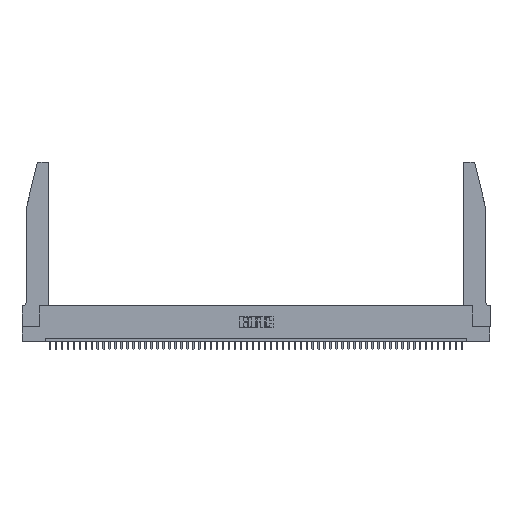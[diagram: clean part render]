
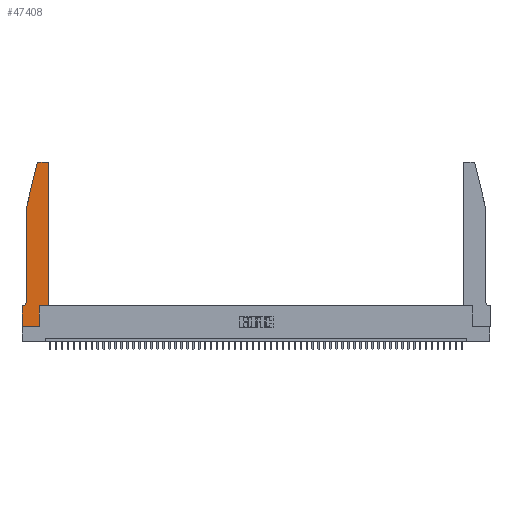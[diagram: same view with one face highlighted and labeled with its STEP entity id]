
A CAD part, top view. The second image highlights one B-rep face of the part: STEP entity #47408.
In plain terms, the highlighted planar face has unit normal (0, 0, 1).
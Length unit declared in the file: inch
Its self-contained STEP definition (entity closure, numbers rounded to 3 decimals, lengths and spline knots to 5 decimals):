
#1088 = VERTEX_POINT ( 'NONE', #7912 ) ;
#1743 = CARTESIAN_POINT ( 'NONE',  ( 0., 0.35, 0.37 ) ) ;
#1959 = VERTEX_POINT ( 'NONE', #51669 ) ;
#2248 = CARTESIAN_POINT ( 'NONE',  ( 0., 0.35, 0.37 ) ) ;
#2281 = CARTESIAN_POINT ( 'NONE',  ( 0.2605, 2.75, 0.37 ) ) ;
#2965 = ORIENTED_EDGE ( 'NONE', *, *, #28072, .T. ) ;
#4232 = VERTEX_POINT ( 'NONE', #18782 ) ;
#4546 = DIRECTION ( 'NONE',  ( -1., 0., 0. ) ) ;
#4662 = ORIENTED_EDGE ( 'NONE', *, *, #48811, .T. ) ;
#4726 = ORIENTED_EDGE ( 'NONE', *, *, #49574, .T. ) ;
#5114 = DIRECTION ( 'NONE',  ( 1., 0., 0. ) ) ;
#5791 = VERTEX_POINT ( 'NONE', #7713 ) ;
#5818 = VECTOR ( 'NONE', #52841, 39.37008 ) ;
#7523 = CARTESIAN_POINT ( 'NONE',  ( 0.4205, 2.75, 0.37 ) ) ;
#7713 = CARTESIAN_POINT ( 'NONE',  ( 0.4505, 2.72, 0.37 ) ) ;
#7912 = CARTESIAN_POINT ( 'NONE',  ( 0., 0., 0.37 ) ) ;
#8651 = LINE ( 'NONE', #51778, #38439 ) ;
#9214 = CARTESIAN_POINT ( 'NONE',  ( 0.25487, 2.72718, 0.37 ) ) ;
#10478 = PLANE ( 'NONE',  #39131 ) ;
#10817 = EDGE_CURVE ( 'NONE', #13678, #48190, #16978, .T. ) ;
#10908 = DIRECTION ( 'NONE',  ( -1., 0., 0. ) ) ;
#12120 = ORIENTED_EDGE ( 'NONE', *, *, #10817, .T. ) ;
#12957 = VERTEX_POINT ( 'NONE', #7523 ) ;
#13678 = VERTEX_POINT ( 'NONE', #21338 ) ;
#14140 = CARTESIAN_POINT ( 'NONE',  ( 0.4505, 0.35, 0.37 ) ) ;
#15595 = ORIENTED_EDGE ( 'NONE', *, *, #46903, .T. ) ;
#15779 = ORIENTED_EDGE ( 'NONE', *, *, #20057, .T. ) ;
#16077 = CARTESIAN_POINT ( 'NONE',  ( 0.4505, 0.35, 0.37 ) ) ;
#16978 = LINE ( 'NONE', #44925, #5818 ) ;
#18343 = VECTOR ( 'NONE', #38082, 39.37008 ) ;
#18782 = CARTESIAN_POINT ( 'NONE',  ( 0.2865, 0.35, 0.37 ) ) ;
#19298 = DIRECTION ( 'NONE',  ( -1., 0., 0. ) ) ;
#20057 = EDGE_CURVE ( 'NONE', #41519, #4232, #24482, .T. ) ;
#20104 = EDGE_CURVE ( 'NONE', #39838, #5791, #31553, .T. ) ;
#21002 = CARTESIAN_POINT ( 'NONE',  ( 0.284, 2.72, 0.37 ) ) ;
#21013 = VERTEX_POINT ( 'NONE', #1743 ) ;
#21338 = CARTESIAN_POINT ( 'NONE',  ( 0.0755, 2., 0.37 ) ) ;
#22242 = ORIENTED_EDGE ( 'NONE', *, *, #29675, .T. ) ;
#23185 = DIRECTION ( 'NONE',  ( 0., 1., 0. ) ) ;
#24482 = LINE ( 'NONE', #29772, #42487 ) ;
#24500 = EDGE_CURVE ( 'NONE', #29545, #13678, #40934, .T. ) ;
#25381 = ORIENTED_EDGE ( 'NONE', *, *, #24500, .T. ) ;
#25647 = ORIENTED_EDGE ( 'NONE', *, *, #41718, .T. ) ;
#26916 = ORIENTED_EDGE ( 'NONE', *, *, #20104, .T. ) ;
#27145 = CARTESIAN_POINT ( 'NONE',  ( 0.4505, 0.35, 0.37 ) ) ;
#28072 = EDGE_CURVE ( 'NONE', #12957, #1959, #34078, .T. ) ;
#29258 = VECTOR ( 'NONE', #5114, 39.37008 ) ;
#29451 = LINE ( 'NONE', #37773, #18343 ) ;
#29545 = VERTEX_POINT ( 'NONE', #9214 ) ;
#29675 = EDGE_CURVE ( 'NONE', #1959, #29545, #45006, .T. ) ;
#29772 = CARTESIAN_POINT ( 'NONE',  ( 0.2865, 0.35, 0.37 ) ) ;
#31260 = EDGE_CURVE ( 'NONE', #1088, #41519, #32553, .T. ) ;
#31553 = LINE ( 'NONE', #14140, #41906 ) ;
#31778 = DIRECTION ( 'NONE',  ( 0., 0., 1. ) ) ;
#32257 = VECTOR ( 'NONE', #10908, 39.37008 ) ;
#32553 = LINE ( 'NONE', #39073, #29258 ) ;
#32842 = DIRECTION ( 'NONE',  ( 0., 0., 1. ) ) ;
#32950 = DIRECTION ( 'NONE',  ( 1., 0., 0. ) ) ;
#33177 = LINE ( 'NONE', #16077, #47219 ) ;
#34078 = LINE ( 'NONE', #2281, #32257 ) ;
#35165 = FACE_OUTER_BOUND ( 'NONE', #35959, .T. ) ;
#35681 = CARTESIAN_POINT ( 'NONE',  ( 0.2865, 0., 0.37 ) ) ;
#35959 = EDGE_LOOP ( 'NONE', ( #2965, #22242, #25381, #12120, #4726, #15595, #42183, #38039, #15779, #4662, #26916, #25647 ) ) ;
#36302 = CIRCLE ( 'NONE', #48580, 0.07 ) ;
#37491 = DIRECTION ( 'NONE',  ( 0., 0., 1. ) ) ;
#37773 = CARTESIAN_POINT ( 'NONE',  ( 0., 0., 0.37 ) ) ;
#37970 = DIRECTION ( 'NONE',  ( 1., 0., 0. ) ) ;
#38039 = ORIENTED_EDGE ( 'NONE', *, *, #31260, .T. ) ;
#38082 = DIRECTION ( 'NONE',  ( 0., -1., 0. ) ) ;
#38439 = VECTOR ( 'NONE', #19298, 39.37008 ) ;
#39073 = CARTESIAN_POINT ( 'NONE',  ( 0., 0., 0.37 ) ) ;
#39131 = AXIS2_PLACEMENT_3D ( 'NONE', #2248, #31778, #52504 ) ;
#39838 = VERTEX_POINT ( 'NONE', #27145 ) ;
#40934 = LINE ( 'NONE', #53039, #44085 ) ;
#41519 = VERTEX_POINT ( 'NONE', #35681 ) ;
#41718 = EDGE_CURVE ( 'NONE', #5791, #12957, #42079, .T. ) ;
#41906 = VECTOR ( 'NONE', #43105, 39.37008 ) ;
#41954 = DIRECTION ( 'NONE',  ( 1., 0., 0. ) ) ;
#42079 = CIRCLE ( 'NONE', #46483, 0.03 ) ;
#42183 = ORIENTED_EDGE ( 'NONE', *, *, #44624, .T. ) ;
#42485 = CARTESIAN_POINT ( 'NONE',  ( 0.0055, 0.35, 0.37 ) ) ;
#42487 = VECTOR ( 'NONE', #23185, 39.37008 ) ;
#43105 = DIRECTION ( 'NONE',  ( 0., 1., 0. ) ) ;
#43445 = VERTEX_POINT ( 'NONE', #42485 ) ;
#44085 = VECTOR ( 'NONE', #52669, 39.37008 ) ;
#44624 = EDGE_CURVE ( 'NONE', #21013, #1088, #29451, .T. ) ;
#44925 = CARTESIAN_POINT ( 'NONE',  ( 0.0755, 2., 0.37 ) ) ;
#45006 = CIRCLE ( 'NONE', #50129, 0.03 ) ;
#45874 = CARTESIAN_POINT ( 'NONE',  ( 0.0055, 0.42, 0.37 ) ) ;
#46039 = CARTESIAN_POINT ( 'NONE',  ( 0.4205, 2.72, 0.37 ) ) ;
#46483 = AXIS2_PLACEMENT_3D ( 'NONE', #46039, #37491, #37970 ) ;
#46903 = EDGE_CURVE ( 'NONE', #43445, #21013, #8651, .T. ) ;
#47219 = VECTOR ( 'NONE', #32950, 39.37008 ) ;
#47408 = ADVANCED_FACE ( 'NONE', ( #35165 ), #10478, .T. ) ;
#48190 = VERTEX_POINT ( 'NONE', #49579 ) ;
#48580 = AXIS2_PLACEMENT_3D ( 'NONE', #45874, #50039, #4546 ) ;
#48811 = EDGE_CURVE ( 'NONE', #4232, #39838, #33177, .T. ) ;
#49574 = EDGE_CURVE ( 'NONE', #48190, #43445, #36302, .T. ) ;
#49579 = CARTESIAN_POINT ( 'NONE',  ( 0.0755, 0.42, 0.37 ) ) ;
#50039 = DIRECTION ( 'NONE',  ( 0., 0., -1. ) ) ;
#50129 = AXIS2_PLACEMENT_3D ( 'NONE', #21002, #32842, #41954 ) ;
#51669 = CARTESIAN_POINT ( 'NONE',  ( 0.284, 2.75, 0.37 ) ) ;
#51778 = CARTESIAN_POINT ( 'NONE',  ( 0.0755, 0.35, 0.37 ) ) ;
#52504 = DIRECTION ( 'NONE',  ( 1., 0., 0. ) ) ;
#52669 = DIRECTION ( 'NONE',  ( -0.239, -0.971, 0. ) ) ;
#52841 = DIRECTION ( 'NONE',  ( 0., -1., 0. ) ) ;
#53039 = CARTESIAN_POINT ( 'NONE',  ( 0.0755, 2., 0.37 ) ) ;
